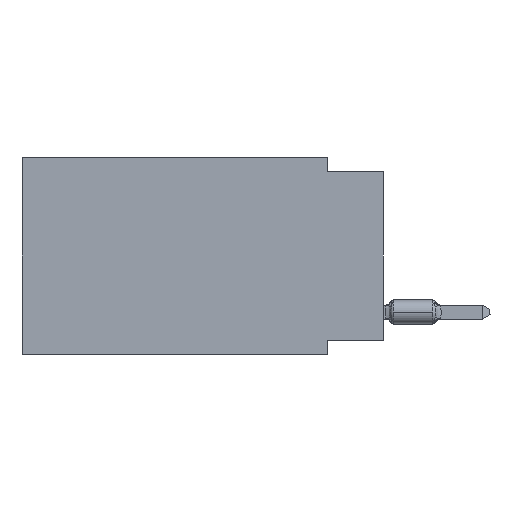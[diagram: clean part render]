
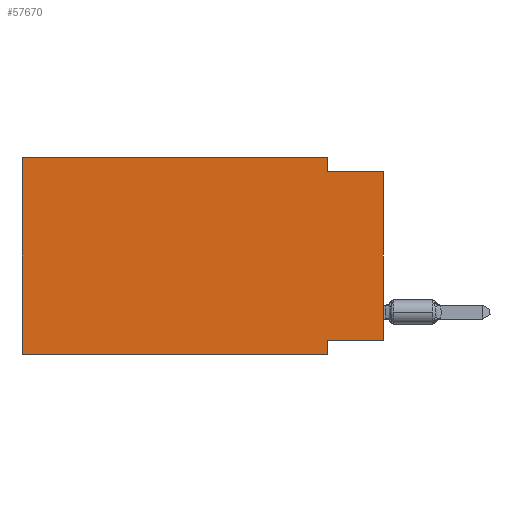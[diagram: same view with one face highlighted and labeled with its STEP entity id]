
A CAD part, left-side view. The second image highlights one B-rep face of the part: STEP entity #57670.
In plain terms, the highlighted planar face has unit normal (-1, 0, 0).
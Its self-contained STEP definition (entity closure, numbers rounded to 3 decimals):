
#157 = CARTESIAN_POINT ( 'NONE',  ( 0., 2.54, 0. ) ) ;
#376 = ORIENTED_EDGE ( 'NONE', *, *, #18643, .F. ) ;
#1611 = PLANE ( 'NONE',  #31191 ) ;
#2788 = EDGE_CURVE ( 'NONE', #62904, #21868, #56703, .T. ) ;
#2821 = VECTOR ( 'NONE', #38004, 1000. ) ;
#5097 = VERTEX_POINT ( 'NONE', #157 ) ;
#5142 = CARTESIAN_POINT ( 'NONE',  ( 0., 16.383, 0. ) ) ;
#5147 = CARTESIAN_POINT ( 'NONE',  ( 0., 16.383, 0. ) ) ;
#5565 = ORIENTED_EDGE ( 'NONE', *, *, #14152, .T. ) ;
#6254 = DIRECTION ( 'NONE',  ( 0., -1., 0. ) ) ;
#8412 = LINE ( 'NONE', #22216, #56956 ) ;
#10009 = VECTOR ( 'NONE', #27874, 1000. ) ;
#10396 = VECTOR ( 'NONE', #39457, 1000. ) ;
#13478 = CARTESIAN_POINT ( 'NONE',  ( 0., 16.383, -8.89 ) ) ;
#13490 = LINE ( 'NONE', #5147, #59865 ) ;
#14049 = VECTOR ( 'NONE', #24724, 1000. ) ;
#14152 = EDGE_CURVE ( 'NONE', #53003, #40863, #52211, .T. ) ;
#14405 = ORIENTED_EDGE ( 'NONE', *, *, #31434, .F. ) ;
#15413 = CARTESIAN_POINT ( 'NONE',  ( 0., 2.54, -8.255 ) ) ;
#15652 = EDGE_LOOP ( 'NONE', ( #36654, #46626, #14405, #37280, #48436, #5565, #376, #29137 ) ) ;
#18643 = EDGE_CURVE ( 'NONE', #21868, #40863, #49358, .T. ) ;
#19809 = CARTESIAN_POINT ( 'NONE',  ( 0., 16.383, -8.89 ) ) ;
#19935 = CARTESIAN_POINT ( 'NONE',  ( 0., 2.54, -8.89 ) ) ;
#20490 = CARTESIAN_POINT ( 'NONE',  ( 0., 16.383, 0. ) ) ;
#20980 = LINE ( 'NONE', #21911, #58701 ) ;
#21868 = VERTEX_POINT ( 'NONE', #15413 ) ;
#21911 = CARTESIAN_POINT ( 'NONE',  ( 0., 16.383, 0. ) ) ;
#22216 = CARTESIAN_POINT ( 'NONE',  ( 0., 0., 0. ) ) ;
#24724 = DIRECTION ( 'NONE',  ( 0., -1., 0. ) ) ;
#25506 = CARTESIAN_POINT ( 'NONE',  ( 0., 0., -0.635 ) ) ;
#25947 = FACE_OUTER_BOUND ( 'NONE', #15652, .T. ) ;
#27332 = DIRECTION ( 'NONE',  ( 0., 0., 1. ) ) ;
#27874 = DIRECTION ( 'NONE',  ( 0., -1., 0. ) ) ;
#29137 = ORIENTED_EDGE ( 'NONE', *, *, #2788, .F. ) ;
#29534 = CARTESIAN_POINT ( 'NONE',  ( 0., 2.54, -0.635 ) ) ;
#31070 = DIRECTION ( 'NONE',  ( 1., 0., 0. ) ) ;
#31191 = AXIS2_PLACEMENT_3D ( 'NONE', #5142, #31070, #31381 ) ;
#31381 = DIRECTION ( 'NONE',  ( 0., 0., -1. ) ) ;
#31434 = EDGE_CURVE ( 'NONE', #5097, #31791, #62625, .T. ) ;
#31791 = VERTEX_POINT ( 'NONE', #29534 ) ;
#32614 = EDGE_CURVE ( 'NONE', #62904, #51442, #8412, .T. ) ;
#35362 = EDGE_CURVE ( 'NONE', #53003, #35962, #13490, .T. ) ;
#35962 = VERTEX_POINT ( 'NONE', #20490 ) ;
#36654 = ORIENTED_EDGE ( 'NONE', *, *, #32614, .T. ) ;
#37280 = ORIENTED_EDGE ( 'NONE', *, *, #57290, .F. ) ;
#38004 = DIRECTION ( 'NONE',  ( 0., 0., -1. ) ) ;
#39457 = DIRECTION ( 'NONE',  ( 0., 0., -1. ) ) ;
#40863 = VERTEX_POINT ( 'NONE', #51318 ) ;
#42810 = CARTESIAN_POINT ( 'NONE',  ( 0., 2.54, 0. ) ) ;
#44228 = LINE ( 'NONE', #54178, #14049 ) ;
#45571 = EDGE_CURVE ( 'NONE', #31791, #51442, #44228, .T. ) ;
#46626 = ORIENTED_EDGE ( 'NONE', *, *, #45571, .F. ) ;
#47378 = CARTESIAN_POINT ( 'NONE',  ( 0., 0., -8.255 ) ) ;
#48436 = ORIENTED_EDGE ( 'NONE', *, *, #35362, .F. ) ;
#48745 = VECTOR ( 'NONE', #57031, 1000. ) ;
#49358 = LINE ( 'NONE', #19935, #10396 ) ;
#51318 = CARTESIAN_POINT ( 'NONE',  ( 0., 2.54, -8.89 ) ) ;
#51442 = VERTEX_POINT ( 'NONE', #25506 ) ;
#52211 = LINE ( 'NONE', #13478, #10009 ) ;
#53003 = VERTEX_POINT ( 'NONE', #19809 ) ;
#54178 = CARTESIAN_POINT ( 'NONE',  ( 0., 0., -0.635 ) ) ;
#56703 = LINE ( 'NONE', #61806, #48745 ) ;
#56956 = VECTOR ( 'NONE', #27332, 1000. ) ;
#57031 = DIRECTION ( 'NONE',  ( 0., 1., 0. ) ) ;
#57290 = EDGE_CURVE ( 'NONE', #35962, #5097, #20980, .T. ) ;
#57670 = ADVANCED_FACE ( 'NONE', ( #25947 ), #1611, .F. ) ;
#58286 = DIRECTION ( 'NONE',  ( 0., 0., 1. ) ) ;
#58701 = VECTOR ( 'NONE', #6254, 1000. ) ;
#59865 = VECTOR ( 'NONE', #58286, 1000. ) ;
#61806 = CARTESIAN_POINT ( 'NONE',  ( 0., 0., -8.255 ) ) ;
#62625 = LINE ( 'NONE', #42810, #2821 ) ;
#62904 = VERTEX_POINT ( 'NONE', #47378 ) ;
